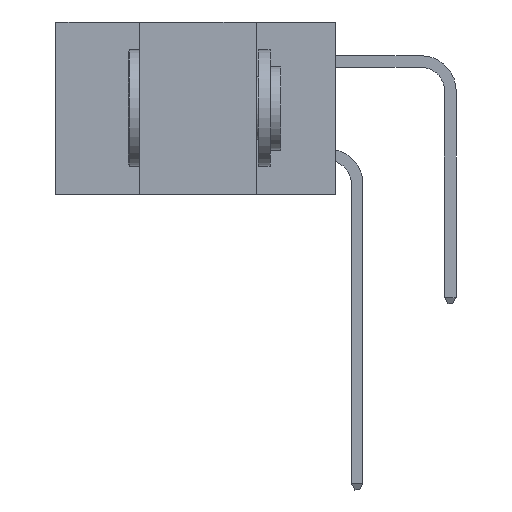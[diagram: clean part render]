
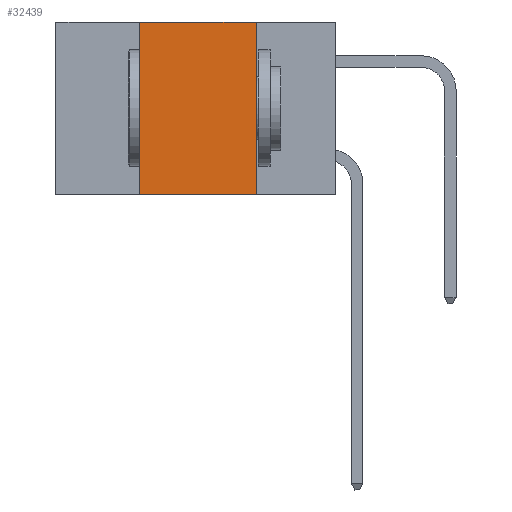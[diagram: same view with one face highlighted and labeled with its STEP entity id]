
A CAD part, left-side view. The second image highlights one B-rep face of the part: STEP entity #32439.
In plain terms, the highlighted planar face has unit normal (-1, 0, 0).
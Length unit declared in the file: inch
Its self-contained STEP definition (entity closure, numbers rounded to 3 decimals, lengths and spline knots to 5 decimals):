
#206 = DIRECTION ( 'NONE',  ( 0., 0., -1. ) ) ;
#856 = VECTOR ( 'NONE', #14196, 39.37008 ) ;
#1203 = LINE ( 'NONE', #14751, #34436 ) ;
#2201 = EDGE_CURVE ( 'NONE', #15689, #7605, #35203, .T. ) ;
#2293 = CARTESIAN_POINT ( 'NONE',  ( 0., 0.6, 0. ) ) ;
#2825 = EDGE_CURVE ( 'NONE', #7605, #2849, #16161, .T. ) ;
#2849 = VERTEX_POINT ( 'NONE', #6223 ) ;
#2938 = VECTOR ( 'NONE', #5127, 39.37008 ) ;
#3477 = ORIENTED_EDGE ( 'NONE', *, *, #2825, .F. ) ;
#5127 = DIRECTION ( 'NONE',  ( 0., -1., 0. ) ) ;
#5914 = EDGE_CURVE ( 'NONE', #14385, #15689, #14142, .T. ) ;
#6223 = CARTESIAN_POINT ( 'NONE',  ( 0., 0.17, -0.37 ) ) ;
#7605 = VERTEX_POINT ( 'NONE', #17669 ) ;
#8313 = DIRECTION ( 'NONE',  ( 0., 0., -1. ) ) ;
#9639 = ORIENTED_EDGE ( 'NONE', *, *, #2201, .F. ) ;
#10575 = AXIS2_PLACEMENT_3D ( 'NONE', #2293, #15291, #8313 ) ;
#10652 = FACE_OUTER_BOUND ( 'NONE', #16711, .T. ) ;
#12087 = CARTESIAN_POINT ( 'NONE',  ( 0., 0.42, 0. ) ) ;
#14142 = LINE ( 'NONE', #32519, #856 ) ;
#14196 = DIRECTION ( 'NONE',  ( 0., 0., 1. ) ) ;
#14385 = VERTEX_POINT ( 'NONE', #38491 ) ;
#14751 = CARTESIAN_POINT ( 'NONE',  ( 0., 0.6, -0.37 ) ) ;
#15291 = DIRECTION ( 'NONE',  ( 1., 0., 0. ) ) ;
#15689 = VERTEX_POINT ( 'NONE', #12087 ) ;
#16161 = LINE ( 'NONE', #24100, #23277 ) ;
#16711 = EDGE_LOOP ( 'NONE', ( #3477, #9639, #27802, #27345 ) ) ;
#17437 = PLANE ( 'NONE',  #10575 ) ;
#17669 = CARTESIAN_POINT ( 'NONE',  ( 0., 0.17, 0. ) ) ;
#20228 = CARTESIAN_POINT ( 'NONE',  ( 0., 0.6, 0. ) ) ;
#23277 = VECTOR ( 'NONE', #206, 39.37008 ) ;
#24100 = CARTESIAN_POINT ( 'NONE',  ( 0., 0.17, 0. ) ) ;
#27345 = ORIENTED_EDGE ( 'NONE', *, *, #30787, .T. ) ;
#27802 = ORIENTED_EDGE ( 'NONE', *, *, #5914, .F. ) ;
#30787 = EDGE_CURVE ( 'NONE', #14385, #2849, #1203, .T. ) ;
#32439 = ADVANCED_FACE ( 'NONE', ( #10652 ), #17437, .F. ) ;
#32519 = CARTESIAN_POINT ( 'NONE',  ( 0., 0.42, 0. ) ) ;
#34436 = VECTOR ( 'NONE', #36003, 39.37008 ) ;
#35203 = LINE ( 'NONE', #20228, #2938 ) ;
#36003 = DIRECTION ( 'NONE',  ( 0., -1., 0. ) ) ;
#38491 = CARTESIAN_POINT ( 'NONE',  ( 0., 0.42, -0.37 ) ) ;
